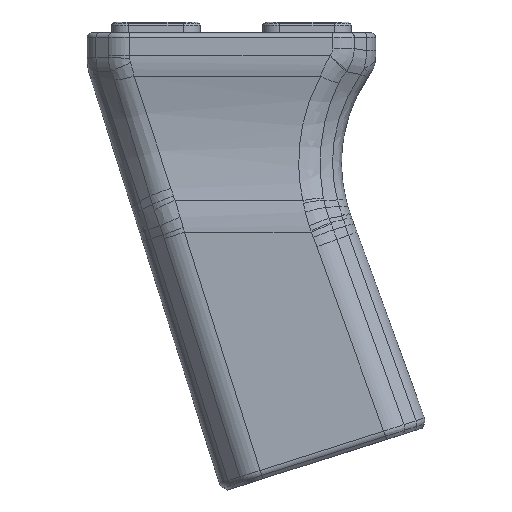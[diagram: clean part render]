
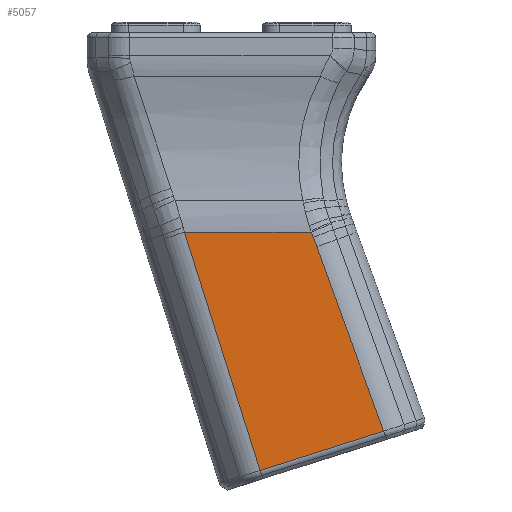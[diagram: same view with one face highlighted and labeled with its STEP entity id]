
A CAD part, left-side view. The second image highlights one B-rep face of the part: STEP entity #5057.
In plain terms, the highlighted planar face has unit normal (-1, 0, 0).
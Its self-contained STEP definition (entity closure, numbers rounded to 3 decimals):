
#115=LINE('',#8590,#357);
#141=LINE('',#9033,#383);
#143=LINE('',#9039,#385);
#144=LINE('',#9050,#386);
#357=VECTOR('',#6059,10.);
#383=VECTOR('',#6195,10.);
#385=VECTOR('',#6201,10.);
#386=VECTOR('',#6202,10.);
#655=PLANE('',#5480);
#832=FACE_OUTER_BOUND('',#1183,.T.);
#1183=EDGE_LOOP('',(#3670,#3671,#3672,#3673,#3674,#3675));
#1510=B_SPLINE_CURVE_WITH_KNOTS('',3,(#9041,#9042,#9043,#9044),
 .UNSPECIFIED.,.F.,.F.,(4,4),(0.,0.133),.UNSPECIFIED.);
#1511=B_SPLINE_CURVE_WITH_KNOTS('',3,(#9046,#9047,#9048,#9049),
 .UNSPECIFIED.,.F.,.F.,(4,4),(0.,0.074),.UNSPECIFIED.);
#2071=VERTEX_POINT('',#8587);
#2072=VERTEX_POINT('',#8589);
#2114=VERTEX_POINT('',#9032);
#2116=VERTEX_POINT('',#9038);
#2117=VERTEX_POINT('',#9040);
#2118=VERTEX_POINT('',#9045);
#2594=EDGE_CURVE('',#2071,#2072,#115,.T.);
#2673=EDGE_CURVE('',#2072,#2114,#141,.T.);
#2676=EDGE_CURVE('',#2116,#2071,#143,.T.);
#2677=EDGE_CURVE('',#2117,#2116,#1510,.T.);
#2678=EDGE_CURVE('',#2118,#2117,#1511,.T.);
#2679=EDGE_CURVE('',#2114,#2118,#144,.T.);
#3670=ORIENTED_EDGE('',*,*,#2594,.F.);
#3671=ORIENTED_EDGE('',*,*,#2676,.F.);
#3672=ORIENTED_EDGE('',*,*,#2677,.F.);
#3673=ORIENTED_EDGE('',*,*,#2678,.F.);
#3674=ORIENTED_EDGE('',*,*,#2679,.F.);
#3675=ORIENTED_EDGE('',*,*,#2673,.F.);
#5057=ADVANCED_FACE('',(#832),#655,.F.);
#5480=AXIS2_PLACEMENT_3D('',#9037,#6199,#6200);
#6059=DIRECTION('',(0.,0.953,-0.303));
#6195=DIRECTION('',(0.,0.303,0.953));
#6199=DIRECTION('center_axis',(1.,0.,0.));
#6200=DIRECTION('ref_axis',(0.,1.,0.));
#6201=DIRECTION('',(0.,-0.341,-0.94));
#6202=DIRECTION('',(0.,-1.,0.));
#8587=CARTESIAN_POINT('',(-10.9,-165.394,50.307));
#8589=CARTESIAN_POINT('',(-10.9,-149.039,45.109));
#8590=CARTESIAN_POINT('',(-10.9,-154.462,46.833));
#9032=CARTESIAN_POINT('',(-10.9,-139.017,76.644));
#9033=CARTESIAN_POINT('',(-10.9,-138.778,77.396));
#9037=CARTESIAN_POINT('Origin',(-10.9,-150.226,72.653));
#9038=CARTESIAN_POINT('',(-10.9,-156.537,74.714));
#9039=CARTESIAN_POINT('',(-10.9,-158.815,68.437));
#9040=CARTESIAN_POINT('',(-10.9,-156.073,75.962));
#9041=CARTESIAN_POINT('Ctrl Pts',(-10.9,-156.073,75.962));
#9042=CARTESIAN_POINT('Ctrl Pts',(-10.9,-156.231,75.547));
#9043=CARTESIAN_POINT('Ctrl Pts',(-10.9,-156.386,75.131));
#9044=CARTESIAN_POINT('Ctrl Pts',(-10.9,-156.537,74.714));
#9045=CARTESIAN_POINT('',(-10.9,-155.799,76.644));
#9046=CARTESIAN_POINT('Ctrl Pts',(-10.9,-155.799,76.644));
#9047=CARTESIAN_POINT('Ctrl Pts',(-10.9,-155.895,76.418));
#9048=CARTESIAN_POINT('Ctrl Pts',(-10.9,-155.986,76.191));
#9049=CARTESIAN_POINT('Ctrl Pts',(-10.9,-156.073,75.962));
#9050=CARTESIAN_POINT('',(-10.9,-164.329,76.644));
